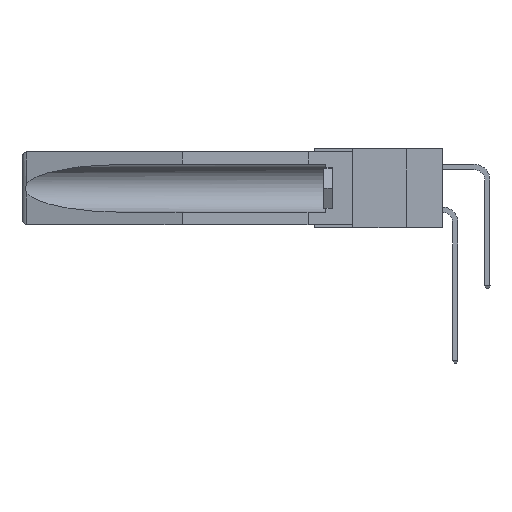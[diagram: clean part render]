
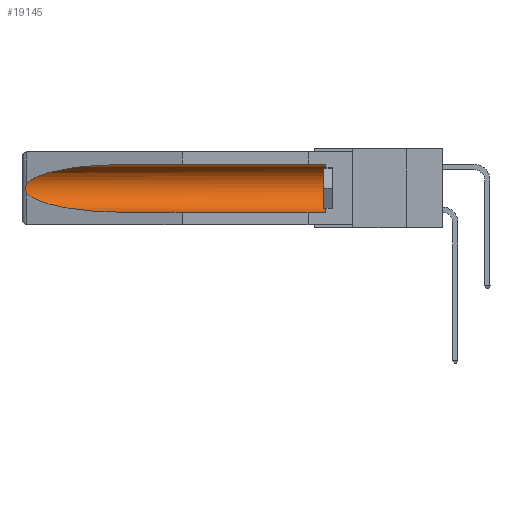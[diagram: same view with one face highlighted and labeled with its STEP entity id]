
A CAD part, left-side view. The second image highlights one B-rep face of the part: STEP entity #19145.
In plain terms, the highlighted cylindrical face has radius 2.857 mm (diameter 5.715 mm), a partial arc.
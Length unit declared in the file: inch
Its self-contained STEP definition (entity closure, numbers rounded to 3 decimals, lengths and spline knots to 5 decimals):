
#253 = CARTESIAN_POINT ( 'NONE',  ( 0.155, 0.126, -0.1715 ) ) ;
#911 = VERTEX_POINT ( 'NONE', #22064 ) ;
#1193 = ORIENTED_EDGE ( 'NONE', *, *, #13026, .T. ) ;
#1551 = CARTESIAN_POINT ( 'NONE',  ( 0.155, 1.07973, -0.059 ) ) ;
#1882 = CARTESIAN_POINT ( 'NONE',  ( 0.155, 0.126, -0.059 ) ) ;
#3533 = AXIS2_PLACEMENT_3D ( 'NONE', #253, #6486, #4283 ) ;
#3995 = CARTESIAN_POINT ( 'NONE',  ( 0.25451, 1.48313, -0.24835 ) ) ;
#4004 = CARTESIAN_POINT ( 'NONE',  ( 0.155, -0.30754, -0.284 ) ) ;
#4283 = DIRECTION ( 'NONE',  ( 0., 0., 1. ) ) ;
#4389 = CARTESIAN_POINT ( 'NONE',  ( 0.26537, 1.52718, -0.14972 ) ) ;
#4479 = CARTESIAN_POINT ( 'NONE',  ( 0.2675, 1.53308, -0.16763 ) ) ;
#4619 = CIRCLE ( 'NONE', #3533, 0.1125 ) ;
#4999 = CARTESIAN_POINT ( 'NONE',  ( 0.155, 1.07973, -0.059 ) ) ;
#5249 = CARTESIAN_POINT ( 'NONE',  ( 0.26537, 1.52718, -0.14972 ) ) ;
#6314 = VECTOR ( 'NONE', #18391, 39.37008 ) ;
#6325 = CARTESIAN_POINT ( 'NONE',  ( 0.26597, 1.52961, -0.15275 ) ) ;
#6484 = ORIENTED_EDGE ( 'NONE', *, *, #15338, .T. ) ;
#6486 = DIRECTION ( 'NONE',  ( 0., -1., 0. ) ) ;
#6501 = CARTESIAN_POINT ( 'NONE',  ( 0.2673, 1.53269, -0.17917 ) ) ;
#6868 = ORIENTED_EDGE ( 'NONE', *, *, #20434, .T. ) ;
#7811 = LINE ( 'NONE', #4004, #12850 ) ;
#7877 = VERTEX_POINT ( 'NONE', #1882 ) ;
#7880 = CARTESIAN_POINT ( 'NONE',  ( 0.21114, 1.30732, -0.059 ) ) ;
#8263 = ORIENTED_EDGE ( 'NONE', *, *, #17253, .F. ) ;
#8680 = VERTEX_POINT ( 'NONE', #14533 ) ;
#9667 = DIRECTION ( 'NONE',  ( 0., 1., 0. ) ) ;
#9872 = CYLINDRICAL_SURFACE ( 'NONE', #25807, 0.1125 ) ;
#10148 = EDGE_CURVE ( 'NONE', #7877, #12846, #25441, .T. ) ;
#10178 = CARTESIAN_POINT ( 'NONE',  ( 0.155, 1.07973, -0.284 ) ) ;
#11092 = EDGE_CURVE ( 'NONE', #911, #24826, #17508, .T. ) ;
#11934 = CARTESIAN_POINT ( 'NONE',  ( 0.25451, 1.48313, -0.09465 ) ) ;
#12337 = CARTESIAN_POINT ( 'NONE',  ( 0.26597, 1.5296, -0.19026 ) ) ;
#12846 = VERTEX_POINT ( 'NONE', #4999 ) ;
#12850 = VECTOR ( 'NONE', #20062, 39.37008 ) ;
#13026 = EDGE_CURVE ( 'NONE', #8680, #7877, #4619, .T. ) ;
#14019 = EDGE_LOOP ( 'NONE', ( #6484, #6868, #21061, #8263, #1193, #14099 ) ) ;
#14099 = ORIENTED_EDGE ( 'NONE', *, *, #10148, .T. ) ;
#14426 = CARTESIAN_POINT ( 'NONE',  ( 0.26654, 1.53092, -0.15636 ) ) ;
#14533 = CARTESIAN_POINT ( 'NONE',  ( 0.155, 0.126, -0.284 ) ) ;
#15338 = EDGE_CURVE ( 'NONE', #12846, #18278, #19904, .T. ) ;
#16566 = DIRECTION ( 'NONE',  ( 0., 0., 1. ) ) ;
#17253 = EDGE_CURVE ( 'NONE', #8680, #24826, #7811, .T. ) ;
#17508 =( BOUNDED_CURVE ( )  B_SPLINE_CURVE ( 3, ( #19529, #3995, #20155, #10178 ),
 .UNSPECIFIED., .F., .F. ) 
 B_SPLINE_CURVE_WITH_KNOTS ( ( 4, 4 ),
 ( 0.1948, 1.5708 ),
 .UNSPECIFIED. ) 
 CURVE ( )  GEOMETRIC_REPRESENTATION_ITEM ( )  RATIONAL_B_SPLINE_CURVE ( ( 1., 0.848, 0.848, 1. ) ) 
 REPRESENTATION_ITEM ( '' )  );
#18119 = CARTESIAN_POINT ( 'NONE',  ( 0.155, 1.07973, -0.284 ) ) ;
#18278 = VERTEX_POINT ( 'NONE', #5249 ) ;
#18391 = DIRECTION ( 'NONE',  ( 0., 1., 0. ) ) ;
#18540 = CARTESIAN_POINT ( 'NONE',  ( 0.26655, 1.53094, -0.18657 ) ) ;
#19145 = ADVANCED_FACE ( 'NONE', ( #23035 ), #9872, .F. ) ;
#19529 = CARTESIAN_POINT ( 'NONE',  ( 0.26537, 1.52718, -0.19328 ) ) ;
#19904 =( BOUNDED_CURVE ( )  B_SPLINE_CURVE ( 3, ( #1551, #7880, #11934, #21887 ),
 .UNSPECIFIED., .F., .F. ) 
 B_SPLINE_CURVE_WITH_KNOTS ( ( 4, 4 ),
 ( 4.71239, 6.08839 ),
 .UNSPECIFIED. ) 
 CURVE ( )  GEOMETRIC_REPRESENTATION_ITEM ( )  RATIONAL_B_SPLINE_CURVE ( ( 1., 0.848, 0.848, 1. ) ) 
 REPRESENTATION_ITEM ( '' )  );
#20062 = DIRECTION ( 'NONE',  ( 0., 1., 0. ) ) ;
#20155 = CARTESIAN_POINT ( 'NONE',  ( 0.21114, 1.30732, -0.284 ) ) ;
#20291 = CARTESIAN_POINT ( 'NONE',  ( 0.26537, 1.52718, -0.19328 ) ) ;
#20434 = EDGE_CURVE ( 'NONE', #18278, #911, #24698, .T. ) ;
#20571 = CARTESIAN_POINT ( 'NONE',  ( 0.155, -0.30754, -0.059 ) ) ;
#21061 = ORIENTED_EDGE ( 'NONE', *, *, #11092, .T. ) ;
#21692 = CARTESIAN_POINT ( 'NONE',  ( 0.155, -0.30754, -0.1715 ) ) ;
#21887 = CARTESIAN_POINT ( 'NONE',  ( 0.26537, 1.52718, -0.14972 ) ) ;
#22064 = CARTESIAN_POINT ( 'NONE',  ( 0.26537, 1.52718, -0.19328 ) ) ;
#22637 = CARTESIAN_POINT ( 'NONE',  ( 0.2673, 1.5327, -0.16383 ) ) ;
#23035 = FACE_OUTER_BOUND ( 'NONE', #14019, .T. ) ;
#24301 = CARTESIAN_POINT ( 'NONE',  ( 0.2675, 1.53308, -0.17534 ) ) ;
#24698 = B_SPLINE_CURVE_WITH_KNOTS ( 'NONE', 3,
 ( #4389, #6325, #14426, #22637, #4479, #24301, #6501, #18540, #12337, #20291 ),
 .UNSPECIFIED., .F., .F.,
 ( 4, 2, 2, 2, 4 ),
 ( 0., 0.00029, 0.00058, 0.00087, 0.00117 ),
 .UNSPECIFIED. ) ;
#24826 = VERTEX_POINT ( 'NONE', #18119 ) ;
#25441 = LINE ( 'NONE', #20571, #6314 ) ;
#25807 = AXIS2_PLACEMENT_3D ( 'NONE', #21692, #9667, #16566 ) ;
